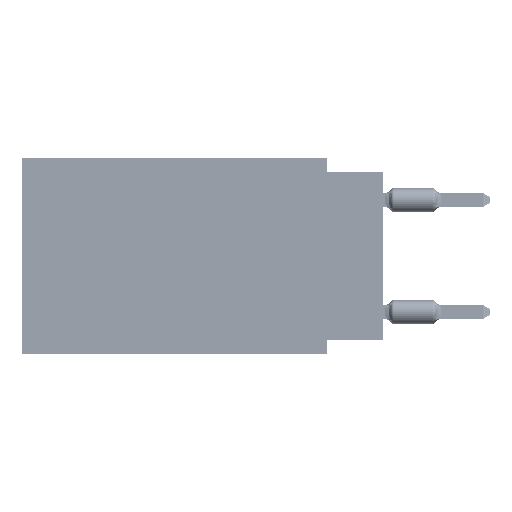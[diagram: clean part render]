
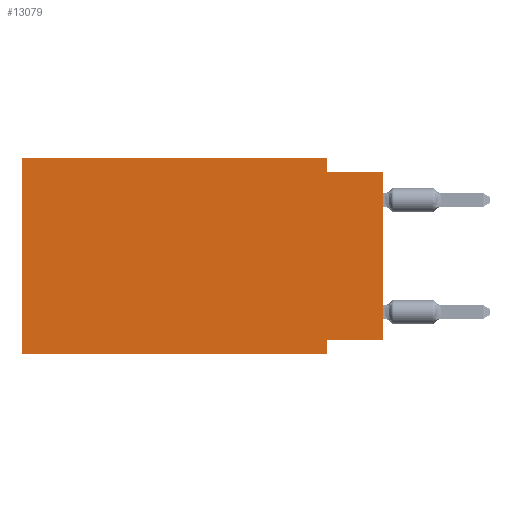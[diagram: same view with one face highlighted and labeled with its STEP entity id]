
A CAD part, left-side view. The second image highlights one B-rep face of the part: STEP entity #13079.
In plain terms, the highlighted planar face has unit normal (-1, 0, 0).
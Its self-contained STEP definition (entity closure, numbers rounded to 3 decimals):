
#133 = PLANE ( 'NONE',  #37957 ) ;
#430 = DIRECTION ( 'NONE',  ( 0., -1., 0. ) ) ;
#2440 = CARTESIAN_POINT ( 'NONE',  ( 0., 2.54, 0. ) ) ;
#5500 = DIRECTION ( 'NONE',  ( 0., 0., -1. ) ) ;
#6309 = EDGE_CURVE ( 'NONE', #39449, #11113, #63487, .T. ) ;
#6484 = DIRECTION ( 'NONE',  ( 0., -1., 0. ) ) ;
#7512 = EDGE_CURVE ( 'NONE', #46246, #61613, #46879, .T. ) ;
#8952 = ORIENTED_EDGE ( 'NONE', *, *, #60102, .F. ) ;
#11113 = VERTEX_POINT ( 'NONE', #18030 ) ;
#13066 = CARTESIAN_POINT ( 'NONE',  ( 0., 16.383, -8.89 ) ) ;
#13079 = ADVANCED_FACE ( 'NONE', ( #30590 ), #133, .F. ) ;
#14905 = DIRECTION ( 'NONE',  ( 0., -1., 0. ) ) ;
#16691 = EDGE_CURVE ( 'NONE', #58453, #56798, #39970, .T. ) ;
#17208 = CARTESIAN_POINT ( 'NONE',  ( 0., 16.383, 0. ) ) ;
#17475 = EDGE_LOOP ( 'NONE', ( #61141, #61680, #53644, #29223, #8952, #57978, #34154, #22766 ) ) ;
#18030 = CARTESIAN_POINT ( 'NONE',  ( 0., 2.54, -8.89 ) ) ;
#18139 = CARTESIAN_POINT ( 'NONE',  ( 0., 0., -0.635 ) ) ;
#18227 = VERTEX_POINT ( 'NONE', #2440 ) ;
#18930 = DIRECTION ( 'NONE',  ( 0., 0., 1. ) ) ;
#21651 = EDGE_CURVE ( 'NONE', #41297, #18227, #22536, .T. ) ;
#22536 = LINE ( 'NONE', #17208, #41885 ) ;
#22766 = ORIENTED_EDGE ( 'NONE', *, *, #7512, .F. ) ;
#24123 = CARTESIAN_POINT ( 'NONE',  ( 0., 2.54, -0.635 ) ) ;
#24995 = EDGE_CURVE ( 'NONE', #18227, #58453, #42450, .T. ) ;
#29223 = ORIENTED_EDGE ( 'NONE', *, *, #21651, .F. ) ;
#30590 = FACE_OUTER_BOUND ( 'NONE', #17475, .T. ) ;
#31430 = VECTOR ( 'NONE', #61407, 1000. ) ;
#31530 = DIRECTION ( 'NONE',  ( 0., 1., 0. ) ) ;
#34154 = ORIENTED_EDGE ( 'NONE', *, *, #48952, .F. ) ;
#36362 = CARTESIAN_POINT ( 'NONE',  ( 0., 16.383, 0. ) ) ;
#37544 = CARTESIAN_POINT ( 'NONE',  ( 0., 0., -8.255 ) ) ;
#37957 = AXIS2_PLACEMENT_3D ( 'NONE', #61629, #54405, #5500 ) ;
#39082 = VECTOR ( 'NONE', #31530, 1000. ) ;
#39449 = VERTEX_POINT ( 'NONE', #45069 ) ;
#39970 = LINE ( 'NONE', #40957, #63689 ) ;
#40208 = VECTOR ( 'NONE', #64957, 1000. ) ;
#40957 = CARTESIAN_POINT ( 'NONE',  ( 0., 0., -0.635 ) ) ;
#41297 = VERTEX_POINT ( 'NONE', #42637 ) ;
#41885 = VECTOR ( 'NONE', #6484, 1000. ) ;
#42450 = LINE ( 'NONE', #42779, #47383 ) ;
#42637 = CARTESIAN_POINT ( 'NONE',  ( 0., 16.383, 0. ) ) ;
#42779 = CARTESIAN_POINT ( 'NONE',  ( 0., 2.54, 0. ) ) ;
#44905 = CARTESIAN_POINT ( 'NONE',  ( 0., 2.54, -8.89 ) ) ;
#45069 = CARTESIAN_POINT ( 'NONE',  ( 0., 16.383, -8.89 ) ) ;
#46246 = VERTEX_POINT ( 'NONE', #51546 ) ;
#46879 = LINE ( 'NONE', #37544, #39082 ) ;
#47383 = VECTOR ( 'NONE', #57785, 1000. ) ;
#48952 = EDGE_CURVE ( 'NONE', #61613, #11113, #54284, .T. ) ;
#50747 = LINE ( 'NONE', #36362, #31430 ) ;
#51546 = CARTESIAN_POINT ( 'NONE',  ( 0., 0., -8.255 ) ) ;
#53430 = EDGE_CURVE ( 'NONE', #46246, #56798, #59314, .T. ) ;
#53644 = ORIENTED_EDGE ( 'NONE', *, *, #24995, .F. ) ;
#54284 = LINE ( 'NONE', #44905, #40208 ) ;
#54405 = DIRECTION ( 'NONE',  ( 1., 0., 0. ) ) ;
#55069 = VECTOR ( 'NONE', #430, 1000. ) ;
#56798 = VERTEX_POINT ( 'NONE', #18139 ) ;
#57785 = DIRECTION ( 'NONE',  ( 0., 0., -1. ) ) ;
#57978 = ORIENTED_EDGE ( 'NONE', *, *, #6309, .T. ) ;
#58453 = VERTEX_POINT ( 'NONE', #24123 ) ;
#59314 = LINE ( 'NONE', #64663, #65029 ) ;
#60102 = EDGE_CURVE ( 'NONE', #39449, #41297, #50747, .T. ) ;
#61141 = ORIENTED_EDGE ( 'NONE', *, *, #53430, .T. ) ;
#61407 = DIRECTION ( 'NONE',  ( 0., 0., 1. ) ) ;
#61613 = VERTEX_POINT ( 'NONE', #62437 ) ;
#61629 = CARTESIAN_POINT ( 'NONE',  ( 0., 16.383, 0. ) ) ;
#61680 = ORIENTED_EDGE ( 'NONE', *, *, #16691, .F. ) ;
#62437 = CARTESIAN_POINT ( 'NONE',  ( 0., 2.54, -8.255 ) ) ;
#63487 = LINE ( 'NONE', #13066, #55069 ) ;
#63689 = VECTOR ( 'NONE', #14905, 1000. ) ;
#64663 = CARTESIAN_POINT ( 'NONE',  ( 0., 0., 0. ) ) ;
#64957 = DIRECTION ( 'NONE',  ( 0., 0., -1. ) ) ;
#65029 = VECTOR ( 'NONE', #18930, 1000. ) ;
